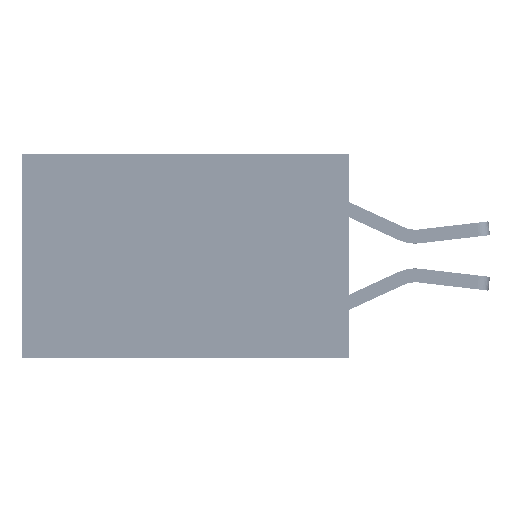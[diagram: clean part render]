
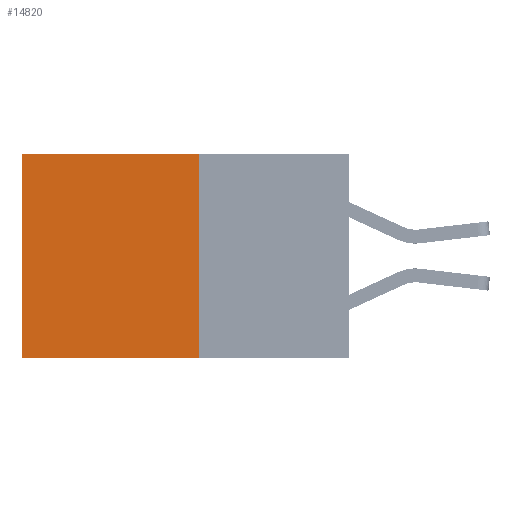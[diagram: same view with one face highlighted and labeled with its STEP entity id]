
A CAD part, left-side view. The second image highlights one B-rep face of the part: STEP entity #14820.
In plain terms, the highlighted planar face has unit normal (-1, 0, 0).
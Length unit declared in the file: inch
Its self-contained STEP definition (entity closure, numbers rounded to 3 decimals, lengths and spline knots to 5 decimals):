
#237 = LINE ( 'NONE', #5870, #27761 ) ;
#294 = VERTEX_POINT ( 'NONE', #16600 ) ;
#849 = LINE ( 'NONE', #16458, #35849 ) ;
#1118 = CARTESIAN_POINT ( 'NONE',  ( 0.277, 0.59, -0.37 ) ) ;
#1125 = CARTESIAN_POINT ( 'NONE',  ( 0.277, 0.27, 0. ) ) ;
#1576 = EDGE_CURVE ( 'NONE', #12744, #14176, #849, .T. ) ;
#1655 = CARTESIAN_POINT ( 'NONE',  ( 0.277, 0.59, 0. ) ) ;
#3479 = DIRECTION ( 'NONE',  ( 0., 1., 0. ) ) ;
#3873 = AXIS2_PLACEMENT_3D ( 'NONE', #15365, #32435, #15610 ) ;
#5870 = CARTESIAN_POINT ( 'NONE',  ( 0.277, 0.59, -0.37 ) ) ;
#7211 = EDGE_CURVE ( 'NONE', #14176, #10770, #237, .T. ) ;
#8364 = DIRECTION ( 'NONE',  ( 0., 0., -1. ) ) ;
#10209 = ORIENTED_EDGE ( 'NONE', *, *, #1576, .T. ) ;
#10391 = ORIENTED_EDGE ( 'NONE', *, *, #7211, .T. ) ;
#10656 = EDGE_CURVE ( 'NONE', #294, #10770, #11649, .T. ) ;
#10770 = VERTEX_POINT ( 'NONE', #1118 ) ;
#11649 = LINE ( 'NONE', #12124, #33282 ) ;
#12124 = CARTESIAN_POINT ( 'NONE',  ( 0.277, 0.27, -0.37 ) ) ;
#12526 = ORIENTED_EDGE ( 'NONE', *, *, #28381, .F. ) ;
#12741 = PLANE ( 'NONE',  #3873 ) ;
#12744 = VERTEX_POINT ( 'NONE', #1125 ) ;
#14176 = VERTEX_POINT ( 'NONE', #1655 ) ;
#14820 = ADVANCED_FACE ( 'NONE', ( #19191 ), #12741, .F. ) ;
#15365 = CARTESIAN_POINT ( 'NONE',  ( 0.277, 0.27, -0.37 ) ) ;
#15610 = DIRECTION ( 'NONE',  ( 0., 0., -1. ) ) ;
#16458 = CARTESIAN_POINT ( 'NONE',  ( 0.277, 0.27, 0. ) ) ;
#16600 = CARTESIAN_POINT ( 'NONE',  ( 0.277, 0.27, -0.37 ) ) ;
#19191 = FACE_OUTER_BOUND ( 'NONE', #31016, .T. ) ;
#20174 = DIRECTION ( 'NONE',  ( 0., 0., -1. ) ) ;
#24127 = ORIENTED_EDGE ( 'NONE', *, *, #10656, .F. ) ;
#25344 = CARTESIAN_POINT ( 'NONE',  ( 0.277, 0.27, -0.37 ) ) ;
#25884 = LINE ( 'NONE', #25344, #26754 ) ;
#26754 = VECTOR ( 'NONE', #8364, 39.37008 ) ;
#27761 = VECTOR ( 'NONE', #20174, 39.37008 ) ;
#28381 = EDGE_CURVE ( 'NONE', #12744, #294, #25884, .T. ) ;
#29009 = DIRECTION ( 'NONE',  ( 0., 1., 0. ) ) ;
#31016 = EDGE_LOOP ( 'NONE', ( #10391, #24127, #12526, #10209 ) ) ;
#32435 = DIRECTION ( 'NONE',  ( 1., 0., 0. ) ) ;
#33282 = VECTOR ( 'NONE', #29009, 39.37008 ) ;
#35849 = VECTOR ( 'NONE', #3479, 39.37008 ) ;
